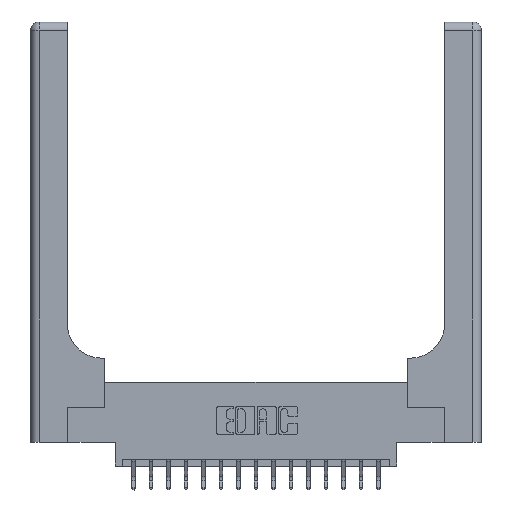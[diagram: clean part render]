
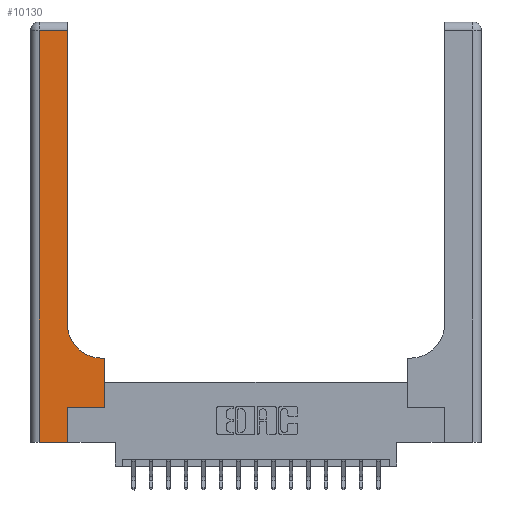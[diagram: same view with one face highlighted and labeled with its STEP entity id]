
A CAD part, top view. The second image highlights one B-rep face of the part: STEP entity #10130.
In plain terms, the highlighted planar face has unit normal (0, 0, 1).
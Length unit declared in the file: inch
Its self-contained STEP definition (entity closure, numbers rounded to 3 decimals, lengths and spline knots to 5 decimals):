
#224 = VECTOR ( 'NONE', #13419, 39.37008 ) ;
#499 = EDGE_CURVE ( 'NONE', #15156, #11073, #2714, .T. ) ;
#1012 = AXIS2_PLACEMENT_3D ( 'NONE', #5885, #16100, #7371 ) ;
#1150 = CARTESIAN_POINT ( 'NONE',  ( 0.06, 3., 0.37 ) ) ;
#1784 = LINE ( 'NONE', #7769, #8754 ) ;
#1853 = CARTESIAN_POINT ( 'NONE',  ( 0.528, 0.25, 0.37 ) ) ;
#2394 = ORIENTED_EDGE ( 'NONE', *, *, #6189, .T. ) ;
#2418 = EDGE_CURVE ( 'NONE', #12541, #5121, #6125, .T. ) ;
#2714 = LINE ( 'NONE', #7317, #17854 ) ;
#2841 = DIRECTION ( 'NONE',  ( 0., 1., 0. ) ) ;
#2888 = PLANE ( 'NONE',  #1012 ) ;
#3274 = EDGE_CURVE ( 'NONE', #4750, #11011, #17742, .T. ) ;
#3608 = CARTESIAN_POINT ( 'NONE',  ( 0., 0., 0.37 ) ) ;
#3609 = CARTESIAN_POINT ( 'NONE',  ( 0.265, 0., 0.37 ) ) ;
#3795 = ORIENTED_EDGE ( 'NONE', *, *, #9689, .T. ) ;
#4160 = LINE ( 'NONE', #11955, #224 ) ;
#4277 = EDGE_CURVE ( 'NONE', #18668, #4750, #4160, .T. ) ;
#4750 = VERTEX_POINT ( 'NONE', #8721 ) ;
#5121 = VERTEX_POINT ( 'NONE', #5538 ) ;
#5178 = CARTESIAN_POINT ( 'NONE',  ( 0.26, 2.94, 0.37 ) ) ;
#5538 = CARTESIAN_POINT ( 'NONE',  ( 0.06, 2.94, 0.37 ) ) ;
#5832 = CARTESIAN_POINT ( 'NONE',  ( 0.06, 0., 0.37 ) ) ;
#5846 = CARTESIAN_POINT ( 'NONE',  ( 0.26, 3., 0.37 ) ) ;
#5885 = CARTESIAN_POINT ( 'NONE',  ( 0., 3., 0.37 ) ) ;
#6125 = LINE ( 'NONE', #7620, #13494 ) ;
#6189 = EDGE_CURVE ( 'NONE', #18417, #15156, #11947, .T. ) ;
#6517 = CARTESIAN_POINT ( 'NONE',  ( 0.26, 0.85, 0.37 ) ) ;
#6535 = EDGE_CURVE ( 'NONE', #5121, #18417, #14225, .T. ) ;
#6610 = DIRECTION ( 'NONE',  ( 1., 0., 0. ) ) ;
#7041 = DIRECTION ( 'NONE',  ( 0., -1., 0. ) ) ;
#7317 = CARTESIAN_POINT ( 'NONE',  ( 0.265, 0., 0.37 ) ) ;
#7357 = DIRECTION ( 'NONE',  ( 0., 1., 0. ) ) ;
#7371 = DIRECTION ( 'NONE',  ( -1., 0., 0. ) ) ;
#7620 = CARTESIAN_POINT ( 'NONE',  ( 0., 2.94, 0.37 ) ) ;
#7769 = CARTESIAN_POINT ( 'NONE',  ( 0.265, 0.25, 0.37 ) ) ;
#7918 = CARTESIAN_POINT ( 'NONE',  ( 0.528, 0.25, 0.37 ) ) ;
#8198 = DIRECTION ( 'NONE',  ( 0., 0., -1. ) ) ;
#8227 = ORIENTED_EDGE ( 'NONE', *, *, #4277, .T. ) ;
#8721 = CARTESIAN_POINT ( 'NONE',  ( 0.51, 0.6, 0.37 ) ) ;
#8754 = VECTOR ( 'NONE', #16501, 39.37008 ) ;
#8864 = LINE ( 'NONE', #5846, #15705 ) ;
#9099 = DIRECTION ( 'NONE',  ( -1., 0., 0. ) ) ;
#9343 = ORIENTED_EDGE ( 'NONE', *, *, #9399, .T. ) ;
#9354 = CARTESIAN_POINT ( 'NONE',  ( 0.528, 0.6, 0.37 ) ) ;
#9399 = EDGE_CURVE ( 'NONE', #11011, #12541, #8864, .T. ) ;
#9591 = CARTESIAN_POINT ( 'NONE',  ( 0.265, 0.25, 0.37 ) ) ;
#9689 = EDGE_CURVE ( 'NONE', #12909, #18668, #11160, .T. ) ;
#10130 = ADVANCED_FACE ( 'NONE', ( #11601 ), #2888, .F. ) ;
#10289 = ORIENTED_EDGE ( 'NONE', *, *, #499, .T. ) ;
#11011 = VERTEX_POINT ( 'NONE', #6517 ) ;
#11073 = VERTEX_POINT ( 'NONE', #9591 ) ;
#11160 = LINE ( 'NONE', #7918, #15024 ) ;
#11601 = FACE_OUTER_BOUND ( 'NONE', #13997, .T. ) ;
#11947 = LINE ( 'NONE', #3608, #15359 ) ;
#11955 = CARTESIAN_POINT ( 'NONE',  ( 0.26, 0.6, 0.37 ) ) ;
#12126 = ORIENTED_EDGE ( 'NONE', *, *, #3274, .T. ) ;
#12541 = VERTEX_POINT ( 'NONE', #5178 ) ;
#12909 = VERTEX_POINT ( 'NONE', #1853 ) ;
#13419 = DIRECTION ( 'NONE',  ( -1., 0., 0. ) ) ;
#13494 = VECTOR ( 'NONE', #9099, 39.37008 ) ;
#13714 = ORIENTED_EDGE ( 'NONE', *, *, #6535, .T. ) ;
#13758 = VECTOR ( 'NONE', #7041, 39.37008 ) ;
#13997 = EDGE_LOOP ( 'NONE', ( #9343, #17099, #13714, #2394, #10289, #18453, #3795, #8227, #12126 ) ) ;
#14225 = LINE ( 'NONE', #1150, #13758 ) ;
#14518 = EDGE_CURVE ( 'NONE', #11073, #12909, #1784, .T. ) ;
#14985 = AXIS2_PLACEMENT_3D ( 'NONE', #16918, #8198, #18368 ) ;
#15024 = VECTOR ( 'NONE', #18094, 39.37008 ) ;
#15156 = VERTEX_POINT ( 'NONE', #3609 ) ;
#15359 = VECTOR ( 'NONE', #6610, 39.37008 ) ;
#15705 = VECTOR ( 'NONE', #2841, 39.37008 ) ;
#16100 = DIRECTION ( 'NONE',  ( 0., 0., -1. ) ) ;
#16501 = DIRECTION ( 'NONE',  ( 1., 0., 0. ) ) ;
#16918 = CARTESIAN_POINT ( 'NONE',  ( 0.51, 0.85, 0.37 ) ) ;
#17099 = ORIENTED_EDGE ( 'NONE', *, *, #2418, .T. ) ;
#17742 = CIRCLE ( 'NONE', #14985, 0.25 ) ;
#17854 = VECTOR ( 'NONE', #7357, 39.37008 ) ;
#18094 = DIRECTION ( 'NONE',  ( 0., 1., 0. ) ) ;
#18368 = DIRECTION ( 'NONE',  ( 1., 0., 0. ) ) ;
#18417 = VERTEX_POINT ( 'NONE', #5832 ) ;
#18453 = ORIENTED_EDGE ( 'NONE', *, *, #14518, .T. ) ;
#18668 = VERTEX_POINT ( 'NONE', #9354 ) ;
